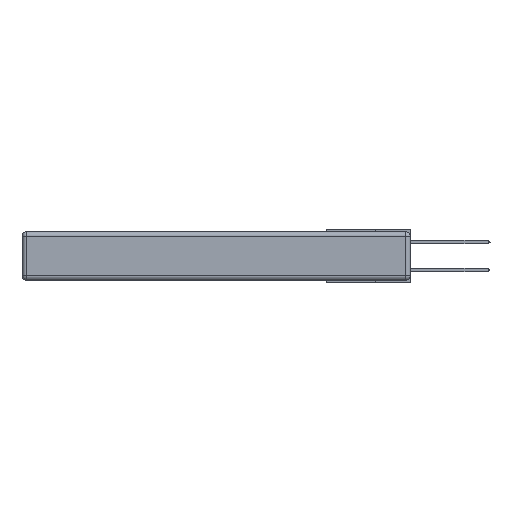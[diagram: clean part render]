
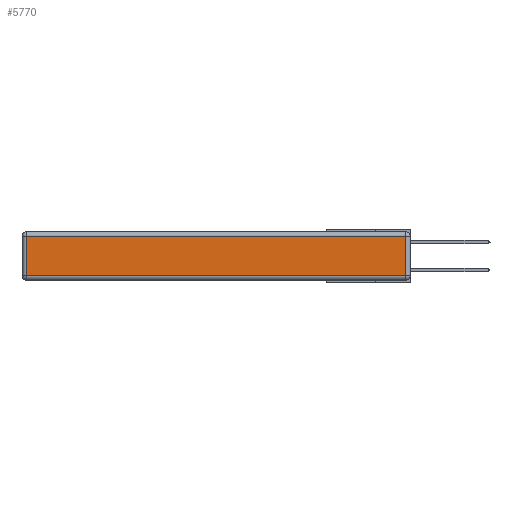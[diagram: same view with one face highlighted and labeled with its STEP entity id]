
A CAD part, left-side view. The second image highlights one B-rep face of the part: STEP entity #5770.
In plain terms, the highlighted planar face has unit normal (-1, 0, 0).
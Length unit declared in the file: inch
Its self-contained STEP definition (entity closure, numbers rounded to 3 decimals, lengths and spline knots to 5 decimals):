
#765 = VECTOR ( 'NONE', #18199, 39.37008 ) ;
#1954 = DIRECTION ( 'NONE',  ( 0., 0., 1. ) ) ;
#2756 = ORIENTED_EDGE ( 'NONE', *, *, #22093, .T. ) ;
#3810 = EDGE_CURVE ( 'NONE', #10619, #16946, #18246, .T. ) ;
#5130 = DIRECTION ( 'NONE',  ( 0., 0., 1. ) ) ;
#5270 = VERTEX_POINT ( 'NONE', #34874 ) ;
#5298 = CARTESIAN_POINT ( 'NONE',  ( 0., 2.72, -0.343 ) ) ;
#5770 = ADVANCED_FACE ( 'NONE', ( #33542 ), #13290, .T. ) ;
#6002 = VECTOR ( 'NONE', #1954, 39.37008 ) ;
#8104 = CARTESIAN_POINT ( 'NONE',  ( 0., 0., -0.313 ) ) ;
#9440 = CARTESIAN_POINT ( 'NONE',  ( 0., 0.03, -0.313 ) ) ;
#10619 = VERTEX_POINT ( 'NONE', #19906 ) ;
#10711 = DIRECTION ( 'NONE',  ( 0., 0., -1. ) ) ;
#13290 = PLANE ( 'NONE',  #29968 ) ;
#14500 = LINE ( 'NONE', #5298, #22966 ) ;
#14570 = VECTOR ( 'NONE', #16787, 39.37008 ) ;
#14996 = LINE ( 'NONE', #34550, #6002 ) ;
#15649 = DIRECTION ( 'NONE',  ( -1., 0., 0. ) ) ;
#16664 = LINE ( 'NONE', #8104, #14570 ) ;
#16787 = DIRECTION ( 'NONE',  ( 0., -1., 0. ) ) ;
#16946 = VERTEX_POINT ( 'NONE', #24971 ) ;
#18199 = DIRECTION ( 'NONE',  ( 0., 1., 0. ) ) ;
#18246 = LINE ( 'NONE', #34565, #765 ) ;
#18732 = CARTESIAN_POINT ( 'NONE',  ( 0., 0., -0.343 ) ) ;
#19906 = CARTESIAN_POINT ( 'NONE',  ( 0., 0.03, -0.03 ) ) ;
#21338 = ORIENTED_EDGE ( 'NONE', *, *, #3810, .T. ) ;
#22093 = EDGE_CURVE ( 'NONE', #16946, #5270, #14500, .T. ) ;
#22641 = ORIENTED_EDGE ( 'NONE', *, *, #33041, .T. ) ;
#22966 = VECTOR ( 'NONE', #10711, 39.37008 ) ;
#24971 = CARTESIAN_POINT ( 'NONE',  ( 0., 2.72, -0.03 ) ) ;
#29303 = EDGE_LOOP ( 'NONE', ( #31946, #22641, #21338, #2756 ) ) ;
#29968 = AXIS2_PLACEMENT_3D ( 'NONE', #18732, #15649, #5130 ) ;
#31946 = ORIENTED_EDGE ( 'NONE', *, *, #33228, .T. ) ;
#33041 = EDGE_CURVE ( 'NONE', #34480, #10619, #14996, .T. ) ;
#33228 = EDGE_CURVE ( 'NONE', #5270, #34480, #16664, .T. ) ;
#33542 = FACE_OUTER_BOUND ( 'NONE', #29303, .T. ) ;
#34480 = VERTEX_POINT ( 'NONE', #9440 ) ;
#34550 = CARTESIAN_POINT ( 'NONE',  ( 0., 0.03, -0.343 ) ) ;
#34565 = CARTESIAN_POINT ( 'NONE',  ( 0., 2.75, -0.03 ) ) ;
#34874 = CARTESIAN_POINT ( 'NONE',  ( 0., 2.72, -0.313 ) ) ;
